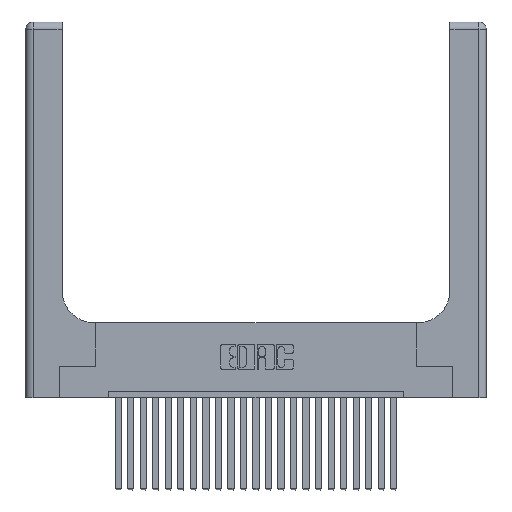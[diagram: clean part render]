
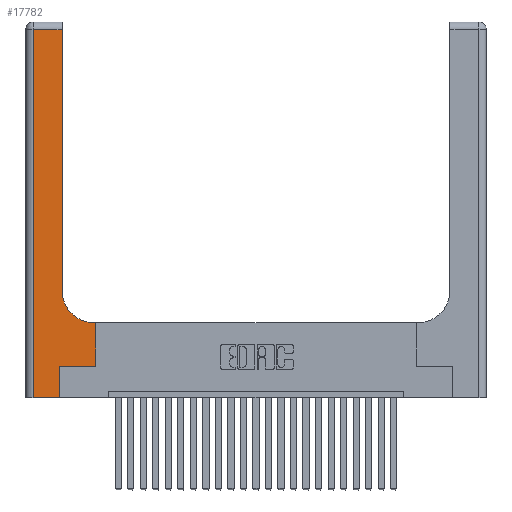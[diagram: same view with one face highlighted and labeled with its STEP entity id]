
A CAD part, top view. The second image highlights one B-rep face of the part: STEP entity #17782.
In plain terms, the highlighted planar face has unit normal (0, 0, 1).
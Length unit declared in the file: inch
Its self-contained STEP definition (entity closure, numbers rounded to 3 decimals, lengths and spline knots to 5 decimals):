
#316 = ORIENTED_EDGE ( 'NONE', *, *, #465, .T. ) ;
#465 = EDGE_CURVE ( 'NONE', #12739, #16947, #7098, .T. ) ;
#1981 = DIRECTION ( 'NONE',  ( 0., 1., 0. ) ) ;
#2154 = LINE ( 'NONE', #19537, #24428 ) ;
#2961 = ORIENTED_EDGE ( 'NONE', *, *, #12390, .T. ) ;
#3121 = VERTEX_POINT ( 'NONE', #19180 ) ;
#3223 = CARTESIAN_POINT ( 'NONE',  ( 0., 0., 0.37 ) ) ;
#3306 = CARTESIAN_POINT ( 'NONE',  ( 0.2915, 3., 0.37 ) ) ;
#3480 = ORIENTED_EDGE ( 'NONE', *, *, #18893, .T. ) ;
#3525 = VECTOR ( 'NONE', #15738, 39.37008 ) ;
#3662 = LINE ( 'NONE', #13460, #12659 ) ;
#4303 = DIRECTION ( 'NONE',  ( 1., 0., 0. ) ) ;
#4363 = FACE_OUTER_BOUND ( 'NONE', #16018, .T. ) ;
#4379 = VECTOR ( 'NONE', #24672, 39.37008 ) ;
#4530 = EDGE_CURVE ( 'NONE', #16947, #12859, #23921, .T. ) ;
#4703 = LINE ( 'NONE', #13074, #4379 ) ;
#5320 = PLANE ( 'NONE',  #20347 ) ;
#5566 = VERTEX_POINT ( 'NONE', #5996 ) ;
#5996 = CARTESIAN_POINT ( 'NONE',  ( 0.5585, 0.25, 0.37 ) ) ;
#6172 = VECTOR ( 'NONE', #24433, 39.37008 ) ;
#6404 = VERTEX_POINT ( 'NONE', #20397 ) ;
#7098 = LINE ( 'NONE', #3306, #22342 ) ;
#7542 = ORIENTED_EDGE ( 'NONE', *, *, #20509, .T. ) ;
#8157 = VECTOR ( 'NONE', #14052, 39.37008 ) ;
#8188 = CARTESIAN_POINT ( 'NONE',  ( 0.5585, 0.25, 0.37 ) ) ;
#8220 = CARTESIAN_POINT ( 'NONE',  ( 0.2915, 2.94, 0.37 ) ) ;
#8437 = LINE ( 'NONE', #8188, #8157 ) ;
#9068 = CARTESIAN_POINT ( 'NONE',  ( 0., 2.94, 0.37 ) ) ;
#9316 = DIRECTION ( 'NONE',  ( -1., 0., 0. ) ) ;
#9441 = AXIS2_PLACEMENT_3D ( 'NONE', #13744, #19457, #4303 ) ;
#9466 = CARTESIAN_POINT ( 'NONE',  ( 0.06, 2.94, 0.37 ) ) ;
#10879 = VERTEX_POINT ( 'NONE', #16624 ) ;
#11239 = DIRECTION ( 'NONE',  ( 0., 0., -1. ) ) ;
#12390 = EDGE_CURVE ( 'NONE', #6404, #15746, #23615, .T. ) ;
#12659 = VECTOR ( 'NONE', #1981, 39.37008 ) ;
#12705 = ORIENTED_EDGE ( 'NONE', *, *, #16565, .T. ) ;
#12739 = VERTEX_POINT ( 'NONE', #15092 ) ;
#12859 = VERTEX_POINT ( 'NONE', #9466 ) ;
#13074 = CARTESIAN_POINT ( 'NONE',  ( 0.06, 3., 0.37 ) ) ;
#13103 = VECTOR ( 'NONE', #18630, 39.37008 ) ;
#13460 = CARTESIAN_POINT ( 'NONE',  ( 0.269, 0., 0.37 ) ) ;
#13744 = CARTESIAN_POINT ( 'NONE',  ( 0.5415, 0.85, 0.37 ) ) ;
#14052 = DIRECTION ( 'NONE',  ( 0., 1., 0. ) ) ;
#15092 = CARTESIAN_POINT ( 'NONE',  ( 0.2915, 0.85, 0.37 ) ) ;
#15205 = VERTEX_POINT ( 'NONE', #19317 ) ;
#15738 = DIRECTION ( 'NONE',  ( -1., 0., 0. ) ) ;
#15746 = VERTEX_POINT ( 'NONE', #22841 ) ;
#15815 = DIRECTION ( 'NONE',  ( 1., 0., 0. ) ) ;
#15914 = ORIENTED_EDGE ( 'NONE', *, *, #19492, .T. ) ;
#16018 = EDGE_LOOP ( 'NONE', ( #316, #19824, #18389, #12705, #15914, #3480, #22939, #2961, #7542 ) ) ;
#16565 = EDGE_CURVE ( 'NONE', #15205, #10879, #23893, .T. ) ;
#16579 = EDGE_CURVE ( 'NONE', #12859, #15205, #4703, .T. ) ;
#16624 = CARTESIAN_POINT ( 'NONE',  ( 0.269, 0., 0.37 ) ) ;
#16947 = VERTEX_POINT ( 'NONE', #8220 ) ;
#17782 = ADVANCED_FACE ( 'NONE', ( #4363 ), #5320, .F. ) ;
#18389 = ORIENTED_EDGE ( 'NONE', *, *, #16579, .T. ) ;
#18630 = DIRECTION ( 'NONE',  ( -1., 0., 0. ) ) ;
#18893 = EDGE_CURVE ( 'NONE', #3121, #5566, #2154, .T. ) ;
#19180 = CARTESIAN_POINT ( 'NONE',  ( 0.269, 0.25, 0.37 ) ) ;
#19317 = CARTESIAN_POINT ( 'NONE',  ( 0.06, 0., 0.37 ) ) ;
#19457 = DIRECTION ( 'NONE',  ( 0., 0., -1. ) ) ;
#19492 = EDGE_CURVE ( 'NONE', #10879, #3121, #3662, .T. ) ;
#19517 = EDGE_CURVE ( 'NONE', #5566, #6404, #8437, .T. ) ;
#19537 = CARTESIAN_POINT ( 'NONE',  ( 0.269, 0.25, 0.37 ) ) ;
#19824 = ORIENTED_EDGE ( 'NONE', *, *, #4530, .T. ) ;
#20347 = AXIS2_PLACEMENT_3D ( 'NONE', #20584, #11239, #9316 ) ;
#20397 = CARTESIAN_POINT ( 'NONE',  ( 0.5585, 0.6, 0.37 ) ) ;
#20434 = CIRCLE ( 'NONE', #9441, 0.25 ) ;
#20509 = EDGE_CURVE ( 'NONE', #15746, #12739, #20434, .T. ) ;
#20584 = CARTESIAN_POINT ( 'NONE',  ( 0., 3., 0.37 ) ) ;
#21057 = CARTESIAN_POINT ( 'NONE',  ( 0.2915, 0.6, 0.37 ) ) ;
#22342 = VECTOR ( 'NONE', #24536, 39.37008 ) ;
#22841 = CARTESIAN_POINT ( 'NONE',  ( 0.5415, 0.6, 0.37 ) ) ;
#22939 = ORIENTED_EDGE ( 'NONE', *, *, #19517, .T. ) ;
#23615 = LINE ( 'NONE', #21057, #3525 ) ;
#23893 = LINE ( 'NONE', #3223, #6172 ) ;
#23921 = LINE ( 'NONE', #9068, #13103 ) ;
#24428 = VECTOR ( 'NONE', #15815, 39.37008 ) ;
#24433 = DIRECTION ( 'NONE',  ( 1., 0., 0. ) ) ;
#24536 = DIRECTION ( 'NONE',  ( 0., 1., 0. ) ) ;
#24672 = DIRECTION ( 'NONE',  ( 0., -1., 0. ) ) ;
